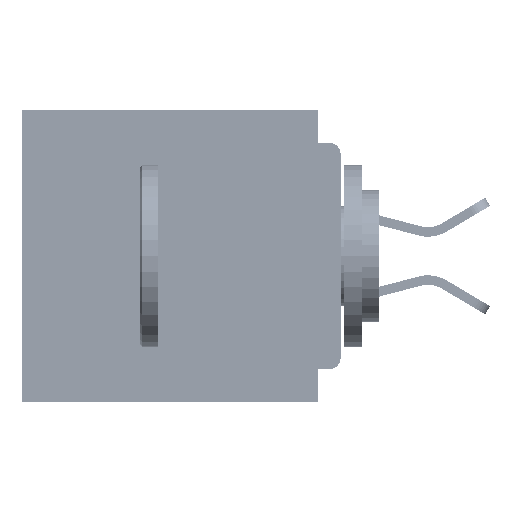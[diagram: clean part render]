
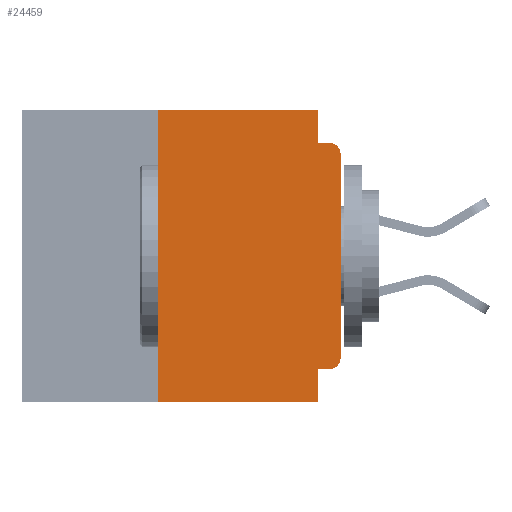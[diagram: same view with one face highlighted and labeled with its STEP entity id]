
A CAD part, left-side view. The second image highlights one B-rep face of the part: STEP entity #24459.
In plain terms, the highlighted planar face has unit normal (-1, 0, 0).
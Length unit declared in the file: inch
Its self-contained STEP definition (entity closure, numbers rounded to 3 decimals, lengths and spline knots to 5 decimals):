
#641 = VERTEX_POINT ( 'NONE', #28151 ) ;
#1358 = DIRECTION ( 'NONE',  ( 0., 0., 1. ) ) ;
#2103 = ORIENTED_EDGE ( 'NONE', *, *, #16511, .T. ) ;
#2766 = EDGE_CURVE ( 'NONE', #67159, #60209, #31278, .T. ) ;
#4441 = CARTESIAN_POINT ( 'NONE',  ( 0., 0.031, -0.4 ) ) ;
#4768 = CARTESIAN_POINT ( 'NONE',  ( 0., 0.015, -0.045 ) ) ;
#7360 = VERTEX_POINT ( 'NONE', #38758 ) ;
#7490 = EDGE_CURVE ( 'NONE', #54126, #7360, #37247, .T. ) ;
#7714 = VERTEX_POINT ( 'NONE', #22054 ) ;
#8706 = VERTEX_POINT ( 'NONE', #4768 ) ;
#9283 = AXIS2_PLACEMENT_3D ( 'NONE', #64951, #64863, #64776 ) ;
#9900 = EDGE_CURVE ( 'NONE', #67159, #52533, #50605, .T. ) ;
#10927 = ORIENTED_EDGE ( 'NONE', *, *, #46735, .F. ) ;
#11696 = ORIENTED_EDGE ( 'NONE', *, *, #7490, .F. ) ;
#11995 = CARTESIAN_POINT ( 'NONE',  ( 0., 0., 0. ) ) ;
#14327 = CARTESIAN_POINT ( 'NONE',  ( 0., 0.437, -0.4 ) ) ;
#14729 = CARTESIAN_POINT ( 'NONE',  ( 0., 0., -0.355 ) ) ;
#16013 = LINE ( 'NONE', #56010, #55867 ) ;
#16511 = EDGE_CURVE ( 'NONE', #60209, #641, #41604, .T. ) ;
#17369 = CARTESIAN_POINT ( 'NONE',  ( 0., 0.25, 0. ) ) ;
#18527 = DIRECTION ( 'NONE',  ( 0., 0., -1. ) ) ;
#18647 = EDGE_CURVE ( 'NONE', #7714, #54126, #56694, .T. ) ;
#19551 = VECTOR ( 'NONE', #55944, 39.37008 ) ;
#19950 = DIRECTION ( 'NONE',  ( 0., 1., 0. ) ) ;
#21217 = LINE ( 'NONE', #14327, #19551 ) ;
#21314 = VECTOR ( 'NONE', #19950, 39.37008 ) ;
#22054 = CARTESIAN_POINT ( 'NONE',  ( 0., 0.25, -0.4 ) ) ;
#24326 = CARTESIAN_POINT ( 'NONE',  ( 0., 0.437, 0. ) ) ;
#24419 = DIRECTION ( 'NONE',  ( 0., 0., 1. ) ) ;
#24459 = ADVANCED_FACE ( 'NONE', ( #57498 ), #44458, .F. ) ;
#25415 = AXIS2_PLACEMENT_3D ( 'NONE', #54704, #49682, #18527 ) ;
#27256 = ORIENTED_EDGE ( 'NONE', *, *, #54167, .T. ) ;
#27644 = VERTEX_POINT ( 'NONE', #40875 ) ;
#28151 = CARTESIAN_POINT ( 'NONE',  ( 0., 0., -0.06 ) ) ;
#28703 = EDGE_LOOP ( 'NONE', ( #2103, #46083, #56799, #10927, #11696, #33087, #27256, #64985, #39335, #42797 ) ) ;
#28785 = VECTOR ( 'NONE', #30512, 39.37008 ) ;
#30512 = DIRECTION ( 'NONE',  ( 0., 0., -1. ) ) ;
#30920 = DIRECTION ( 'NONE',  ( -1., 0., 0. ) ) ;
#30922 = DIRECTION ( 'NONE',  ( 0., 0., -1. ) ) ;
#31278 = CIRCLE ( 'NONE', #9283, 0.015 ) ;
#32179 = EDGE_CURVE ( 'NONE', #52533, #27644, #56419, .T. ) ;
#33087 = ORIENTED_EDGE ( 'NONE', *, *, #18647, .F. ) ;
#36611 = CIRCLE ( 'NONE', #37610, 0.015 ) ;
#37247 = LINE ( 'NONE', #24326, #63139 ) ;
#37610 = AXIS2_PLACEMENT_3D ( 'NONE', #61951, #30920, #67148 ) ;
#37987 = VERTEX_POINT ( 'NONE', #61738 ) ;
#38758 = CARTESIAN_POINT ( 'NONE',  ( 0., 0.031, 0. ) ) ;
#39335 = ORIENTED_EDGE ( 'NONE', *, *, #9900, .F. ) ;
#40061 = CARTESIAN_POINT ( 'NONE',  ( 0., 0., -0.34 ) ) ;
#40875 = CARTESIAN_POINT ( 'NONE',  ( 0., 0.031, -0.4 ) ) ;
#41287 = VECTOR ( 'NONE', #24419, 39.37008 ) ;
#41604 = LINE ( 'NONE', #11995, #53814 ) ;
#41723 = EDGE_CURVE ( 'NONE', #37987, #8706, #16013, .T. ) ;
#42797 = ORIENTED_EDGE ( 'NONE', *, *, #2766, .T. ) ;
#44458 = PLANE ( 'NONE',  #25415 ) ;
#46083 = ORIENTED_EDGE ( 'NONE', *, *, #66917, .T. ) ;
#46735 = EDGE_CURVE ( 'NONE', #7360, #37987, #50183, .T. ) ;
#49682 = DIRECTION ( 'NONE',  ( 1., 0., 0. ) ) ;
#50183 = LINE ( 'NONE', #67151, #62296 ) ;
#50280 = DIRECTION ( 'NONE',  ( 0., -1., 0. ) ) ;
#50605 = LINE ( 'NONE', #14729, #21314 ) ;
#52533 = VERTEX_POINT ( 'NONE', #61820 ) ;
#53408 = CARTESIAN_POINT ( 'NONE',  ( 0., 0.015, -0.355 ) ) ;
#53814 = VECTOR ( 'NONE', #1358, 39.37008 ) ;
#54126 = VERTEX_POINT ( 'NONE', #17369 ) ;
#54167 = EDGE_CURVE ( 'NONE', #7714, #27644, #21217, .T. ) ;
#54704 = CARTESIAN_POINT ( 'NONE',  ( 0., 0.437, 0. ) ) ;
#55867 = VECTOR ( 'NONE', #61187, 39.37008 ) ;
#55944 = DIRECTION ( 'NONE',  ( 0., -1., 0. ) ) ;
#56010 = CARTESIAN_POINT ( 'NONE',  ( 0., 0., -0.045 ) ) ;
#56419 = LINE ( 'NONE', #4441, #28785 ) ;
#56694 = LINE ( 'NONE', #60747, #41287 ) ;
#56799 = ORIENTED_EDGE ( 'NONE', *, *, #41723, .F. ) ;
#57498 = FACE_OUTER_BOUND ( 'NONE', #28703, .T. ) ;
#60209 = VERTEX_POINT ( 'NONE', #40061 ) ;
#60747 = CARTESIAN_POINT ( 'NONE',  ( 0., 0.25, -0.4 ) ) ;
#61187 = DIRECTION ( 'NONE',  ( 0., -1., 0. ) ) ;
#61738 = CARTESIAN_POINT ( 'NONE',  ( 0., 0.031, -0.045 ) ) ;
#61820 = CARTESIAN_POINT ( 'NONE',  ( 0., 0.031, -0.355 ) ) ;
#61951 = CARTESIAN_POINT ( 'NONE',  ( 0., 0.015, -0.06 ) ) ;
#62296 = VECTOR ( 'NONE', #30922, 39.37008 ) ;
#63139 = VECTOR ( 'NONE', #50280, 39.37008 ) ;
#64776 = DIRECTION ( 'NONE',  ( 0., 0., -1. ) ) ;
#64863 = DIRECTION ( 'NONE',  ( -1., 0., 0. ) ) ;
#64951 = CARTESIAN_POINT ( 'NONE',  ( 0., 0.015, -0.34 ) ) ;
#64985 = ORIENTED_EDGE ( 'NONE', *, *, #32179, .F. ) ;
#66917 = EDGE_CURVE ( 'NONE', #641, #8706, #36611, .T. ) ;
#67148 = DIRECTION ( 'NONE',  ( 0., 0., -1. ) ) ;
#67151 = CARTESIAN_POINT ( 'NONE',  ( 0., 0.031, 0. ) ) ;
#67159 = VERTEX_POINT ( 'NONE', #53408 ) ;
